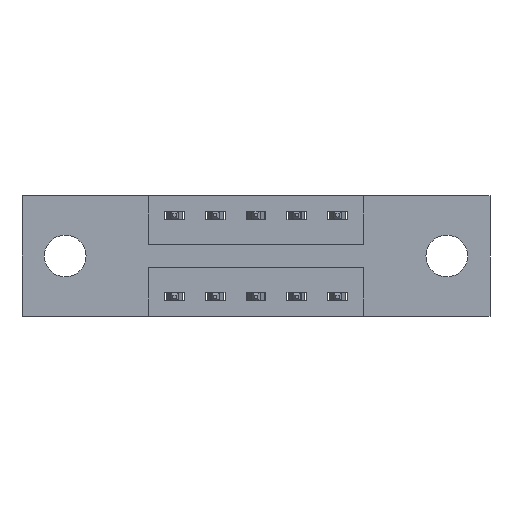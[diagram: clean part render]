
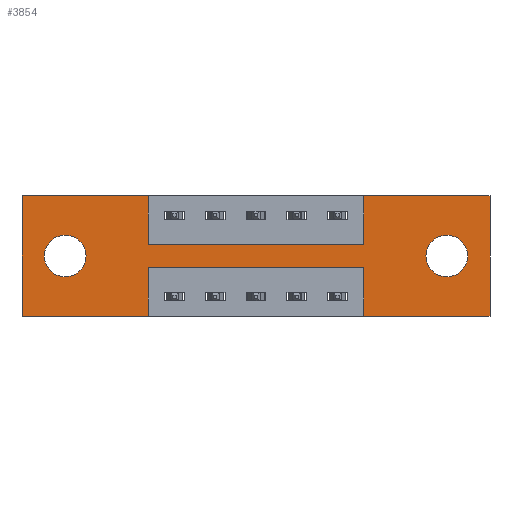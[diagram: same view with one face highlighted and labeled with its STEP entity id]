
A CAD part, front view. The second image highlights one B-rep face of the part: STEP entity #3854.
In plain terms, the highlighted planar face has unit normal (0, -1, 0).
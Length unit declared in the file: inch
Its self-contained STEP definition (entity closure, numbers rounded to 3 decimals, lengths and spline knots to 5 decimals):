
#1 = CARTESIAN_POINT ( 'NONE',  ( 0.3875, 0., -0.37 ) ) ;
#20 = LINE ( 'NONE', #397, #1979 ) ;
#62 = DIRECTION ( 'NONE',  ( 0., 0., -1. ) ) ;
#100 = CARTESIAN_POINT ( 'NONE',  ( 1.3025, 0., -0.185 ) ) ;
#240 = VECTOR ( 'NONE', #4465, 39.37008 ) ;
#348 = ORIENTED_EDGE ( 'NONE', *, *, #4373, .F. ) ;
#397 = CARTESIAN_POINT ( 'NONE',  ( 0.3875, 0., 0. ) ) ;
#423 = VECTOR ( 'NONE', #4833, 39.37008 ) ;
#445 = ORIENTED_EDGE ( 'NONE', *, *, #1329, .F. ) ;
#453 = ORIENTED_EDGE ( 'NONE', *, *, #4803, .T. ) ;
#481 = VERTEX_POINT ( 'NONE', #2848 ) ;
#516 = VERTEX_POINT ( 'NONE', #3470 ) ;
#664 = DIRECTION ( 'NONE',  ( 0., 0., 1. ) ) ;
#671 = VECTOR ( 'NONE', #6964, 39.37008 ) ;
#707 = FACE_BOUND ( 'NONE', #1130, .T. ) ;
#768 = AXIS2_PLACEMENT_3D ( 'NONE', #6112, #2835, #6748 ) ;
#844 = EDGE_CURVE ( 'NONE', #481, #4188, #6717, .T. ) ;
#856 = DIRECTION ( 'NONE',  ( 0., 0., 1. ) ) ;
#956 = VECTOR ( 'NONE', #856, 39.37008 ) ;
#1123 = CARTESIAN_POINT ( 'NONE',  ( 0., 0., 0. ) ) ;
#1126 = ORIENTED_EDGE ( 'NONE', *, *, #2499, .F. ) ;
#1128 = CARTESIAN_POINT ( 'NONE',  ( 0.3875, 0., -0.15 ) ) ;
#1130 = EDGE_LOOP ( 'NONE', ( #4847, #8177 ) ) ;
#1201 = EDGE_CURVE ( 'NONE', #5097, #481, #8076, .T. ) ;
#1218 = EDGE_CURVE ( 'NONE', #2401, #4140, #4994, .T. ) ;
#1304 = AXIS2_PLACEMENT_3D ( 'NONE', #100, #3299, #7120 ) ;
#1329 = EDGE_CURVE ( 'NONE', #4188, #4777, #3883, .T. ) ;
#1374 = AXIS2_PLACEMENT_3D ( 'NONE', #7528, #1753, #1810 ) ;
#1395 = VERTEX_POINT ( 'NONE', #4431 ) ;
#1450 = CARTESIAN_POINT ( 'NONE',  ( 0.3875, 0., -0.37 ) ) ;
#1752 = ORIENTED_EDGE ( 'NONE', *, *, #844, .F. ) ;
#1753 = DIRECTION ( 'NONE',  ( 0., 1., 0. ) ) ;
#1761 = CARTESIAN_POINT ( 'NONE',  ( 0.1325, 0., -0.121 ) ) ;
#1776 = DIRECTION ( 'NONE',  ( 1., 0., 0. ) ) ;
#1810 = DIRECTION ( 'NONE',  ( 0., 0., 1. ) ) ;
#1855 = CARTESIAN_POINT ( 'NONE',  ( 0., 0., -0.37 ) ) ;
#1894 = CARTESIAN_POINT ( 'NONE',  ( 1.0475, 0., 0. ) ) ;
#1931 = EDGE_CURVE ( 'NONE', #4848, #5087, #3575, .T. ) ;
#1964 = ORIENTED_EDGE ( 'NONE', *, *, #2511, .F. ) ;
#1979 = VECTOR ( 'NONE', #5513, 39.37008 ) ;
#1980 = ORIENTED_EDGE ( 'NONE', *, *, #4827, .F. ) ;
#2074 = VECTOR ( 'NONE', #1776, 39.37008 ) ;
#2209 = PLANE ( 'NONE',  #2600 ) ;
#2302 = CARTESIAN_POINT ( 'NONE',  ( 1.0475, 0., -0.37 ) ) ;
#2335 = ORIENTED_EDGE ( 'NONE', *, *, #7719, .F. ) ;
#2337 = CARTESIAN_POINT ( 'NONE',  ( 1.435, 0., -0.37 ) ) ;
#2395 = LINE ( 'NONE', #1128, #4778 ) ;
#2401 = VERTEX_POINT ( 'NONE', #4918 ) ;
#2499 = EDGE_CURVE ( 'NONE', #516, #5794, #2395, .T. ) ;
#2511 = EDGE_CURVE ( 'NONE', #7715, #6181, #4677, .T. ) ;
#2512 = VECTOR ( 'NONE', #6864, 39.37008 ) ;
#2600 = AXIS2_PLACEMENT_3D ( 'NONE', #4756, #2878, #2797 ) ;
#2734 = LINE ( 'NONE', #1123, #5117 ) ;
#2797 = DIRECTION ( 'NONE',  ( 0., 0., -1. ) ) ;
#2835 = DIRECTION ( 'NONE',  ( 0., 1., 0. ) ) ;
#2843 = CARTESIAN_POINT ( 'NONE',  ( 0.3875, 0., 0. ) ) ;
#2848 = CARTESIAN_POINT ( 'NONE',  ( 0.3875, 0., -0.22 ) ) ;
#2868 = LINE ( 'NONE', #7455, #2074 ) ;
#2878 = DIRECTION ( 'NONE',  ( 0., -1., 0. ) ) ;
#2988 = EDGE_CURVE ( 'NONE', #7244, #516, #20, .T. ) ;
#3145 = EDGE_CURVE ( 'NONE', #5794, #1395, #7361, .T. ) ;
#3225 = ORIENTED_EDGE ( 'NONE', *, *, #2988, .F. ) ;
#3229 = LINE ( 'NONE', #5910, #956 ) ;
#3299 = DIRECTION ( 'NONE',  ( 0., 1., 0. ) ) ;
#3310 = EDGE_CURVE ( 'NONE', #4777, #5551, #3229, .T. ) ;
#3418 = CARTESIAN_POINT ( 'NONE',  ( 0., 0., 0. ) ) ;
#3470 = CARTESIAN_POINT ( 'NONE',  ( 0.3875, 0., -0.15 ) ) ;
#3508 = ORIENTED_EDGE ( 'NONE', *, *, #1201, .F. ) ;
#3575 = CIRCLE ( 'NONE', #1304, 0.064 ) ;
#3643 = LINE ( 'NONE', #5769, #240 ) ;
#3663 = DIRECTION ( 'NONE',  ( 1., 0., 0. ) ) ;
#3784 = CARTESIAN_POINT ( 'NONE',  ( 1.0475, 0., -0.22 ) ) ;
#3854 = ADVANCED_FACE ( 'NONE', ( #6337, #707, #4222 ), #2209, .T. ) ;
#3883 = LINE ( 'NONE', #6232, #2512 ) ;
#3929 = VECTOR ( 'NONE', #664, 39.37008 ) ;
#3958 = DIRECTION ( 'NONE',  ( 0., 1., 0. ) ) ;
#4019 = CARTESIAN_POINT ( 'NONE',  ( 1.3025, 0., -0.249 ) ) ;
#4059 = CIRCLE ( 'NONE', #5753, 0.064 ) ;
#4140 = VERTEX_POINT ( 'NONE', #1761 ) ;
#4188 = VERTEX_POINT ( 'NONE', #1450 ) ;
#4222 = FACE_OUTER_BOUND ( 'NONE', #6900, .T. ) ;
#4327 = DIRECTION ( 'NONE',  ( 1., 0., 0. ) ) ;
#4373 = EDGE_CURVE ( 'NONE', #1395, #5895, #2868, .T. ) ;
#4431 = CARTESIAN_POINT ( 'NONE',  ( 1.0475, 0., 0. ) ) ;
#4433 = CIRCLE ( 'NONE', #1374, 0.064 ) ;
#4465 = DIRECTION ( 'NONE',  ( 0., 0., -1. ) ) ;
#4533 = CARTESIAN_POINT ( 'NONE',  ( 1.0475, 0., -0.15 ) ) ;
#4646 = CARTESIAN_POINT ( 'NONE',  ( 1.3025, 0., -0.185 ) ) ;
#4677 = LINE ( 'NONE', #1855, #671 ) ;
#4756 = CARTESIAN_POINT ( 'NONE',  ( 0., 0., -0.37 ) ) ;
#4777 = VERTEX_POINT ( 'NONE', #5273 ) ;
#4778 = VECTOR ( 'NONE', #4327, 39.37008 ) ;
#4803 = EDGE_CURVE ( 'NONE', #5087, #4848, #4059, .T. ) ;
#4827 = EDGE_CURVE ( 'NONE', #5895, #7715, #3643, .T. ) ;
#4833 = DIRECTION ( 'NONE',  ( 0., 0., 1. ) ) ;
#4843 = DIRECTION ( 'NONE',  ( -1., 0., 0. ) ) ;
#4847 = ORIENTED_EDGE ( 'NONE', *, *, #4952, .T. ) ;
#4848 = VERTEX_POINT ( 'NONE', #4019 ) ;
#4918 = CARTESIAN_POINT ( 'NONE',  ( 0.1325, 0., -0.249 ) ) ;
#4952 = EDGE_CURVE ( 'NONE', #4140, #2401, #4433, .T. ) ;
#4973 = ORIENTED_EDGE ( 'NONE', *, *, #5115, .F. ) ;
#4994 = CIRCLE ( 'NONE', #768, 0.064 ) ;
#5086 = ORIENTED_EDGE ( 'NONE', *, *, #3310, .F. ) ;
#5087 = VERTEX_POINT ( 'NONE', #8165 ) ;
#5097 = VERTEX_POINT ( 'NONE', #3784 ) ;
#5115 = EDGE_CURVE ( 'NONE', #6181, #5097, #7810, .T. ) ;
#5117 = VECTOR ( 'NONE', #3663, 39.37008 ) ;
#5273 = CARTESIAN_POINT ( 'NONE',  ( 0., 0., -0.37 ) ) ;
#5513 = DIRECTION ( 'NONE',  ( 0., 0., -1. ) ) ;
#5551 = VERTEX_POINT ( 'NONE', #3418 ) ;
#5562 = ORIENTED_EDGE ( 'NONE', *, *, #3145, .F. ) ;
#5753 = AXIS2_PLACEMENT_3D ( 'NONE', #4646, #3958, #7140 ) ;
#5769 = CARTESIAN_POINT ( 'NONE',  ( 1.435, 0., 0. ) ) ;
#5794 = VERTEX_POINT ( 'NONE', #4533 ) ;
#5895 = VERTEX_POINT ( 'NONE', #7732 ) ;
#5910 = CARTESIAN_POINT ( 'NONE',  ( 0., 0., 0. ) ) ;
#5996 = VECTOR ( 'NONE', #4843, 39.37008 ) ;
#6079 = CARTESIAN_POINT ( 'NONE',  ( 0.3875, 0., -0.22 ) ) ;
#6112 = CARTESIAN_POINT ( 'NONE',  ( 0.1325, 0., -0.185 ) ) ;
#6181 = VERTEX_POINT ( 'NONE', #2302 ) ;
#6232 = CARTESIAN_POINT ( 'NONE',  ( 0., 0., -0.37 ) ) ;
#6337 = FACE_BOUND ( 'NONE', #7328, .T. ) ;
#6507 = VECTOR ( 'NONE', #62, 39.37008 ) ;
#6717 = LINE ( 'NONE', #1, #6507 ) ;
#6748 = DIRECTION ( 'NONE',  ( 0., 0., 1. ) ) ;
#6864 = DIRECTION ( 'NONE',  ( -1., 0., 0. ) ) ;
#6900 = EDGE_LOOP ( 'NONE', ( #1752, #3508, #4973, #1964, #1980, #348, #5562, #1126, #3225, #2335, #5086, #445 ) ) ;
#6964 = DIRECTION ( 'NONE',  ( -1., 0., 0. ) ) ;
#7120 = DIRECTION ( 'NONE',  ( 0., 0., -1. ) ) ;
#7140 = DIRECTION ( 'NONE',  ( 0., 0., -1. ) ) ;
#7244 = VERTEX_POINT ( 'NONE', #2843 ) ;
#7291 = ORIENTED_EDGE ( 'NONE', *, *, #1931, .T. ) ;
#7328 = EDGE_LOOP ( 'NONE', ( #453, #7291 ) ) ;
#7361 = LINE ( 'NONE', #1894, #3929 ) ;
#7455 = CARTESIAN_POINT ( 'NONE',  ( 0., 0., 0. ) ) ;
#7528 = CARTESIAN_POINT ( 'NONE',  ( 0.1325, 0., -0.185 ) ) ;
#7715 = VERTEX_POINT ( 'NONE', #2337 ) ;
#7719 = EDGE_CURVE ( 'NONE', #5551, #7244, #2734, .T. ) ;
#7732 = CARTESIAN_POINT ( 'NONE',  ( 1.435, 0., 0. ) ) ;
#7810 = LINE ( 'NONE', #7999, #423 ) ;
#7999 = CARTESIAN_POINT ( 'NONE',  ( 1.0475, 0., -0.37 ) ) ;
#8076 = LINE ( 'NONE', #6079, #5996 ) ;
#8165 = CARTESIAN_POINT ( 'NONE',  ( 1.3025, 0., -0.121 ) ) ;
#8177 = ORIENTED_EDGE ( 'NONE', *, *, #1218, .T. ) ;
